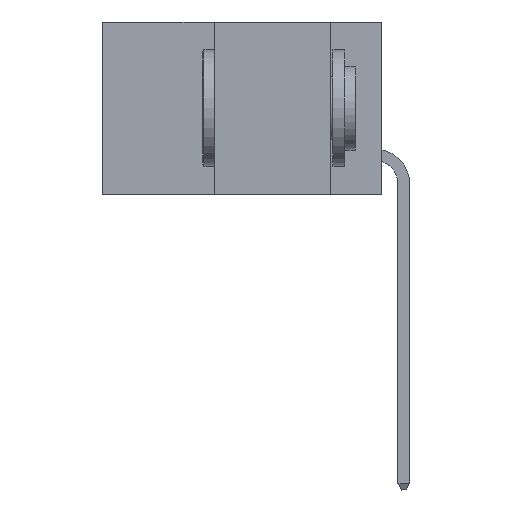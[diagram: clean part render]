
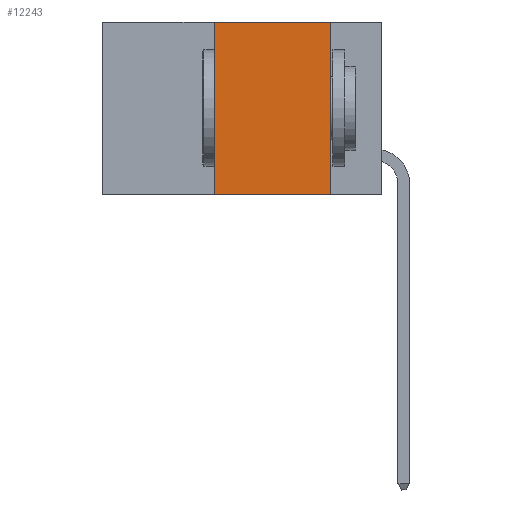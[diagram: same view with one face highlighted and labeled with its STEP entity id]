
A CAD part, left-side view. The second image highlights one B-rep face of the part: STEP entity #12243.
In plain terms, the highlighted planar face has unit normal (-1, 0, 0).
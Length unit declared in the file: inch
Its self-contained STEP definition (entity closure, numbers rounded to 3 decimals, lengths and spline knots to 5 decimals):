
#237 = LINE ( 'NONE', #2286, #1935 ) ;
#737 = CARTESIAN_POINT ( 'NONE',  ( 0., 0.36, -0.37 ) ) ;
#1935 = VECTOR ( 'NONE', #5302, 39.37008 ) ;
#2059 = VECTOR ( 'NONE', #2085, 39.37008 ) ;
#2085 = DIRECTION ( 'NONE',  ( 0., 0., 1. ) ) ;
#2286 = CARTESIAN_POINT ( 'NONE',  ( 0., 0.6, -0.37 ) ) ;
#2559 = ORIENTED_EDGE ( 'NONE', *, *, #18677, .F. ) ;
#3173 = CARTESIAN_POINT ( 'NONE',  ( 0., 0.11, 0. ) ) ;
#4612 = CARTESIAN_POINT ( 'NONE',  ( 0., 0.11, 0. ) ) ;
#4830 = EDGE_CURVE ( 'NONE', #13889, #11706, #237, .T. ) ;
#5302 = DIRECTION ( 'NONE',  ( 0., -1., 0. ) ) ;
#6028 = LINE ( 'NONE', #3173, #10387 ) ;
#6173 = LINE ( 'NONE', #6674, #2059 ) ;
#6674 = CARTESIAN_POINT ( 'NONE',  ( 0., 0.36, 0. ) ) ;
#6864 = VERTEX_POINT ( 'NONE', #4612 ) ;
#8860 = ORIENTED_EDGE ( 'NONE', *, *, #11630, .F. ) ;
#9806 = CARTESIAN_POINT ( 'NONE',  ( 0., 0.36, 0. ) ) ;
#10344 = ORIENTED_EDGE ( 'NONE', *, *, #11629, .F. ) ;
#10387 = VECTOR ( 'NONE', #14710, 39.37008 ) ;
#11629 = EDGE_CURVE ( 'NONE', #6864, #11706, #6028, .T. ) ;
#11630 = EDGE_CURVE ( 'NONE', #17728, #6864, #19172, .T. ) ;
#11706 = VERTEX_POINT ( 'NONE', #13978 ) ;
#11783 = ORIENTED_EDGE ( 'NONE', *, *, #4830, .T. ) ;
#12243 = ADVANCED_FACE ( 'NONE', ( #18179 ), #13627, .F. ) ;
#12783 = CARTESIAN_POINT ( 'NONE',  ( 0., 0.6, 0. ) ) ;
#13627 = PLANE ( 'NONE',  #17281 ) ;
#13889 = VERTEX_POINT ( 'NONE', #737 ) ;
#13978 = CARTESIAN_POINT ( 'NONE',  ( 0., 0.11, -0.37 ) ) ;
#14129 = CARTESIAN_POINT ( 'NONE',  ( 0., 0.6, 0. ) ) ;
#14710 = DIRECTION ( 'NONE',  ( 0., 0., -1. ) ) ;
#16852 = DIRECTION ( 'NONE',  ( 0., 0., -1. ) ) ;
#17281 = AXIS2_PLACEMENT_3D ( 'NONE', #14129, #18789, #16852 ) ;
#17728 = VERTEX_POINT ( 'NONE', #9806 ) ;
#18179 = FACE_OUTER_BOUND ( 'NONE', #18531, .T. ) ;
#18531 = EDGE_LOOP ( 'NONE', ( #10344, #8860, #2559, #11783 ) ) ;
#18677 = EDGE_CURVE ( 'NONE', #13889, #17728, #6173, .T. ) ;
#18789 = DIRECTION ( 'NONE',  ( 1., 0., 0. ) ) ;
#19172 = LINE ( 'NONE', #12783, #19896 ) ;
#19303 = DIRECTION ( 'NONE',  ( 0., -1., 0. ) ) ;
#19896 = VECTOR ( 'NONE', #19303, 39.37008 ) ;
